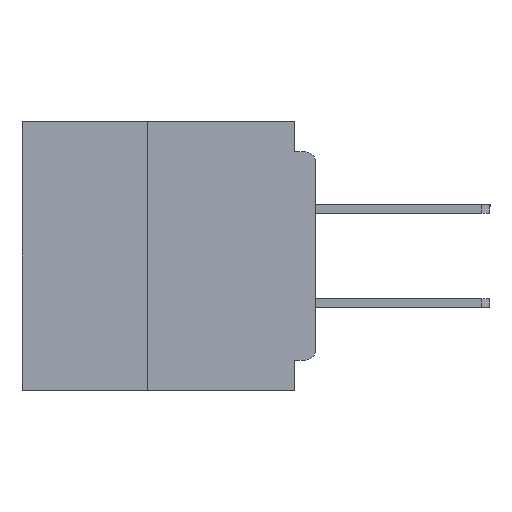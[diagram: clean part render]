
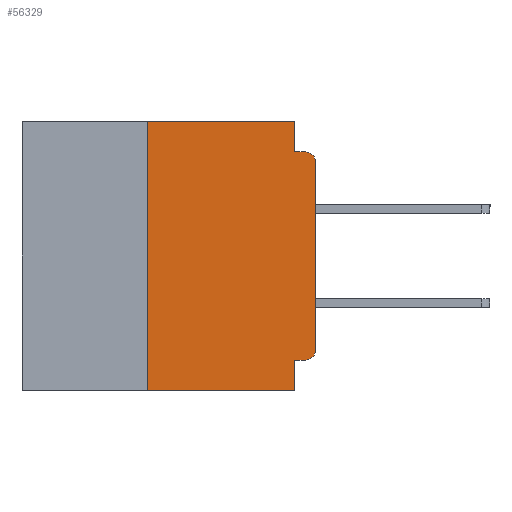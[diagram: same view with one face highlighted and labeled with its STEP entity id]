
A CAD part, left-side view. The second image highlights one B-rep face of the part: STEP entity #56329.
In plain terms, the highlighted planar face has unit normal (-1, 0, 0).
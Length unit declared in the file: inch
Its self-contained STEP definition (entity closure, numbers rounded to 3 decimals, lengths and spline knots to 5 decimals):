
#109 = CIRCLE ( 'NONE', #60131, 0.015 ) ;
#262 = ORIENTED_EDGE ( 'NONE', *, *, #18191, .F. ) ;
#734 = ORIENTED_EDGE ( 'NONE', *, *, #37212, .T. ) ;
#1244 = CARTESIAN_POINT ( 'NONE',  ( 0., 0., -0.34 ) ) ;
#2604 = VERTEX_POINT ( 'NONE', #30705 ) ;
#4158 = EDGE_CURVE ( 'NONE', #63909, #34963, #34755, .T. ) ;
#4420 = CIRCLE ( 'NONE', #24147, 0.015 ) ;
#7697 = CARTESIAN_POINT ( 'NONE',  ( 0., 0.031, 0. ) ) ;
#7869 = CARTESIAN_POINT ( 'NONE',  ( 0., 0.031, -0.355 ) ) ;
#10060 = DIRECTION ( 'NONE',  ( 0., 0., -1. ) ) ;
#10184 = CARTESIAN_POINT ( 'NONE',  ( 0., 0.015, -0.045 ) ) ;
#10984 = VERTEX_POINT ( 'NONE', #10184 ) ;
#11249 = VECTOR ( 'NONE', #41464, 39.37008 ) ;
#11446 = AXIS2_PLACEMENT_3D ( 'NONE', #57436, #52447, #21548 ) ;
#12505 = LINE ( 'NONE', #20105, #65864 ) ;
#13325 = CARTESIAN_POINT ( 'NONE',  ( 0., 0., -0.06 ) ) ;
#14645 = VECTOR ( 'NONE', #15780, 39.37008 ) ;
#15780 = DIRECTION ( 'NONE',  ( 0., 0., 1. ) ) ;
#16251 = DIRECTION ( 'NONE',  ( -1., 0., 0. ) ) ;
#16528 = EDGE_CURVE ( 'NONE', #34963, #2604, #23730, .T. ) ;
#17432 = FACE_OUTER_BOUND ( 'NONE', #59074, .T. ) ;
#17523 = VERTEX_POINT ( 'NONE', #13325 ) ;
#17742 = VECTOR ( 'NONE', #54257, 39.37008 ) ;
#18191 = EDGE_CURVE ( 'NONE', #58623, #64389, #19201, .T. ) ;
#19201 = LINE ( 'NONE', #34593, #43443 ) ;
#19384 = ORIENTED_EDGE ( 'NONE', *, *, #40059, .F. ) ;
#20105 = CARTESIAN_POINT ( 'NONE',  ( 0., 0.437, -0.4 ) ) ;
#20505 = ORIENTED_EDGE ( 'NONE', *, *, #53737, .F. ) ;
#21331 = PLANE ( 'NONE',  #11446 ) ;
#21548 = DIRECTION ( 'NONE',  ( 0., 0., -1. ) ) ;
#22668 = CARTESIAN_POINT ( 'NONE',  ( 0., 0.031, -0.045 ) ) ;
#23730 = LINE ( 'NONE', #28967, #37503 ) ;
#24147 = AXIS2_PLACEMENT_3D ( 'NONE', #47223, #16251, #52382 ) ;
#28041 = CARTESIAN_POINT ( 'NONE',  ( 0., 0.25, -0.4 ) ) ;
#28684 = ORIENTED_EDGE ( 'NONE', *, *, #4158, .F. ) ;
#28967 = CARTESIAN_POINT ( 'NONE',  ( 0., 0.031, -0.4 ) ) ;
#30705 = CARTESIAN_POINT ( 'NONE',  ( 0., 0.031, -0.4 ) ) ;
#30765 = CARTESIAN_POINT ( 'NONE',  ( 0., 0.031, 0. ) ) ;
#30848 = DIRECTION ( 'NONE',  ( -1., 0., 0. ) ) ;
#31240 = CARTESIAN_POINT ( 'NONE',  ( 0., 0., 0. ) ) ;
#32053 = CARTESIAN_POINT ( 'NONE',  ( 0., 0.25, 0. ) ) ;
#33141 = VECTOR ( 'NONE', #44046, 39.37008 ) ;
#33937 = CARTESIAN_POINT ( 'NONE',  ( 0., 0., -0.355 ) ) ;
#34593 = CARTESIAN_POINT ( 'NONE',  ( 0., 0.25, -0.4 ) ) ;
#34755 = LINE ( 'NONE', #33937, #33141 ) ;
#34804 = LINE ( 'NONE', #49093, #17742 ) ;
#34963 = VERTEX_POINT ( 'NONE', #7869 ) ;
#35298 = ORIENTED_EDGE ( 'NONE', *, *, #54071, .F. ) ;
#35696 = CARTESIAN_POINT ( 'NONE',  ( 0., 0.015, -0.355 ) ) ;
#36301 = CARTESIAN_POINT ( 'NONE',  ( 0., 0.437, 0. ) ) ;
#36643 = VERTEX_POINT ( 'NONE', #1244 ) ;
#36890 = ORIENTED_EDGE ( 'NONE', *, *, #39426, .T. ) ;
#37212 = EDGE_CURVE ( 'NONE', #63909, #36643, #4420, .T. ) ;
#37503 = VECTOR ( 'NONE', #65026, 39.37008 ) ;
#38868 = LINE ( 'NONE', #36301, #11249 ) ;
#39121 = VERTEX_POINT ( 'NONE', #7697 ) ;
#39426 = EDGE_CURVE ( 'NONE', #17523, #10984, #109, .T. ) ;
#40059 = EDGE_CURVE ( 'NONE', #39121, #57995, #57592, .T. ) ;
#40649 = VECTOR ( 'NONE', #10060, 39.37008 ) ;
#41464 = DIRECTION ( 'NONE',  ( 0., -1., 0. ) ) ;
#42184 = LINE ( 'NONE', #31240, #14645 ) ;
#43185 = ORIENTED_EDGE ( 'NONE', *, *, #51549, .T. ) ;
#43443 = VECTOR ( 'NONE', #60267, 39.37008 ) ;
#43864 = ORIENTED_EDGE ( 'NONE', *, *, #16528, .F. ) ;
#44046 = DIRECTION ( 'NONE',  ( 0., 1., 0. ) ) ;
#47223 = CARTESIAN_POINT ( 'NONE',  ( 0., 0.015, -0.34 ) ) ;
#49093 = CARTESIAN_POINT ( 'NONE',  ( 0., 0., -0.045 ) ) ;
#49696 = EDGE_CURVE ( 'NONE', #58623, #2604, #12505, .T. ) ;
#51026 = DIRECTION ( 'NONE',  ( 0., -1., 0. ) ) ;
#51549 = EDGE_CURVE ( 'NONE', #36643, #17523, #42184, .T. ) ;
#52382 = DIRECTION ( 'NONE',  ( 0., 0., -1. ) ) ;
#52447 = DIRECTION ( 'NONE',  ( 1., 0., 0. ) ) ;
#53737 = EDGE_CURVE ( 'NONE', #64389, #39121, #38868, .T. ) ;
#54071 = EDGE_CURVE ( 'NONE', #57995, #10984, #34804, .T. ) ;
#54257 = DIRECTION ( 'NONE',  ( 0., -1., 0. ) ) ;
#56329 = ADVANCED_FACE ( 'NONE', ( #17432 ), #21331, .F. ) ;
#57436 = CARTESIAN_POINT ( 'NONE',  ( 0., 0.437, 0. ) ) ;
#57592 = LINE ( 'NONE', #30765, #40649 ) ;
#57995 = VERTEX_POINT ( 'NONE', #22668 ) ;
#58623 = VERTEX_POINT ( 'NONE', #28041 ) ;
#59074 = EDGE_LOOP ( 'NONE', ( #43185, #36890, #35298, #19384, #20505, #262, #66775, #43864, #28684, #734 ) ) ;
#60131 = AXIS2_PLACEMENT_3D ( 'NONE', #61713, #30848, #66873 ) ;
#60267 = DIRECTION ( 'NONE',  ( 0., 0., 1. ) ) ;
#61713 = CARTESIAN_POINT ( 'NONE',  ( 0., 0.015, -0.06 ) ) ;
#63909 = VERTEX_POINT ( 'NONE', #35696 ) ;
#64389 = VERTEX_POINT ( 'NONE', #32053 ) ;
#65026 = DIRECTION ( 'NONE',  ( 0., 0., -1. ) ) ;
#65864 = VECTOR ( 'NONE', #51026, 39.37008 ) ;
#66775 = ORIENTED_EDGE ( 'NONE', *, *, #49696, .T. ) ;
#66873 = DIRECTION ( 'NONE',  ( 0., 0., -1. ) ) ;
